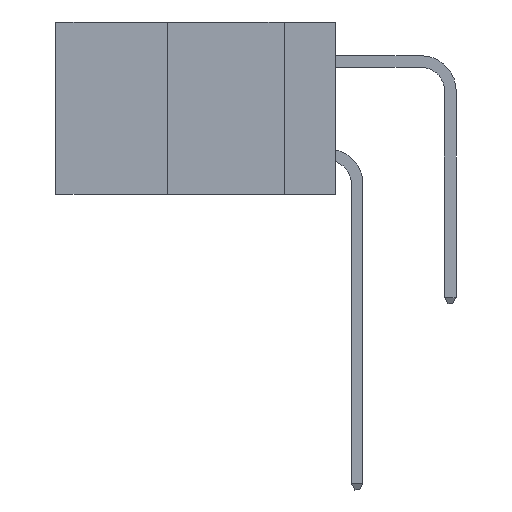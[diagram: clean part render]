
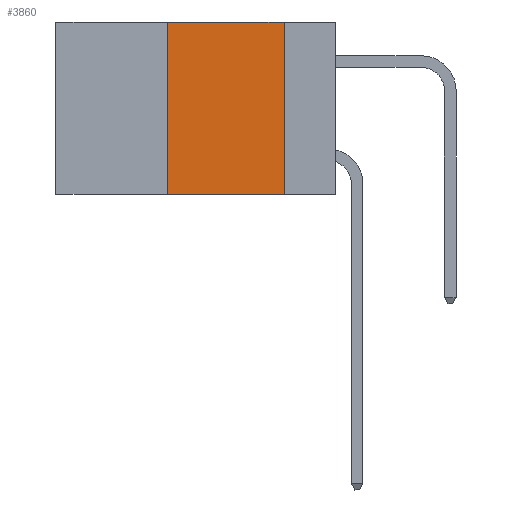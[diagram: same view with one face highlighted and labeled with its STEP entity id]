
A CAD part, left-side view. The second image highlights one B-rep face of the part: STEP entity #3860.
In plain terms, the highlighted planar face has unit normal (-1, 0, 0).
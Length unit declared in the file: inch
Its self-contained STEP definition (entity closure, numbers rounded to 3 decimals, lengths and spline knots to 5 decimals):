
#208 = EDGE_CURVE ( 'NONE', #9338, #5126, #3238, .T. ) ;
#663 = VECTOR ( 'NONE', #11545, 39.37008 ) ;
#905 = VERTEX_POINT ( 'NONE', #10213 ) ;
#1512 = DIRECTION ( 'NONE',  ( 1., 0., 0. ) ) ;
#1621 = EDGE_CURVE ( 'NONE', #6237, #5126, #12207, .T. ) ;
#3238 = LINE ( 'NONE', #8236, #6260 ) ;
#3373 = CARTESIAN_POINT ( 'NONE',  ( 0., 0.36, -0.37 ) ) ;
#3453 = AXIS2_PLACEMENT_3D ( 'NONE', #5565, #1512, #9603 ) ;
#3673 = PLANE ( 'NONE',  #3453 ) ;
#3782 = VECTOR ( 'NONE', #8217, 39.37008 ) ;
#3860 = ADVANCED_FACE ( 'NONE', ( #10355 ), #3673, .F. ) ;
#3988 = CARTESIAN_POINT ( 'NONE',  ( 0., 0.11, 0. ) ) ;
#4109 = CARTESIAN_POINT ( 'NONE',  ( 0., 0.6, 0. ) ) ;
#4140 = EDGE_CURVE ( 'NONE', #905, #9338, #12769, .T. ) ;
#4694 = ORIENTED_EDGE ( 'NONE', *, *, #208, .F. ) ;
#5126 = VERTEX_POINT ( 'NONE', #11727 ) ;
#5190 = CARTESIAN_POINT ( 'NONE',  ( 0., 0.36, 0. ) ) ;
#5565 = CARTESIAN_POINT ( 'NONE',  ( 0., 0.6, 0. ) ) ;
#6237 = VERTEX_POINT ( 'NONE', #3373 ) ;
#6260 = VECTOR ( 'NONE', #6440, 39.37008 ) ;
#6440 = DIRECTION ( 'NONE',  ( 0., 0., -1. ) ) ;
#6964 = ORIENTED_EDGE ( 'NONE', *, *, #1621, .T. ) ;
#8217 = DIRECTION ( 'NONE',  ( 0., -1., 0. ) ) ;
#8236 = CARTESIAN_POINT ( 'NONE',  ( 0., 0.11, 0. ) ) ;
#8338 = ORIENTED_EDGE ( 'NONE', *, *, #10442, .F. ) ;
#9298 = EDGE_LOOP ( 'NONE', ( #4694, #9344, #8338, #6964 ) ) ;
#9338 = VERTEX_POINT ( 'NONE', #3988 ) ;
#9344 = ORIENTED_EDGE ( 'NONE', *, *, #4140, .F. ) ;
#9603 = DIRECTION ( 'NONE',  ( 0., 0., -1. ) ) ;
#10213 = CARTESIAN_POINT ( 'NONE',  ( 0., 0.36, 0. ) ) ;
#10355 = FACE_OUTER_BOUND ( 'NONE', #9298, .T. ) ;
#10442 = EDGE_CURVE ( 'NONE', #6237, #905, #11769, .T. ) ;
#10535 = CARTESIAN_POINT ( 'NONE',  ( 0., 0.6, -0.37 ) ) ;
#10632 = DIRECTION ( 'NONE',  ( 0., -1., 0. ) ) ;
#11068 = VECTOR ( 'NONE', #10632, 39.37008 ) ;
#11545 = DIRECTION ( 'NONE',  ( 0., 0., 1. ) ) ;
#11727 = CARTESIAN_POINT ( 'NONE',  ( 0., 0.11, -0.37 ) ) ;
#11769 = LINE ( 'NONE', #5190, #663 ) ;
#12207 = LINE ( 'NONE', #10535, #11068 ) ;
#12769 = LINE ( 'NONE', #4109, #3782 ) ;
